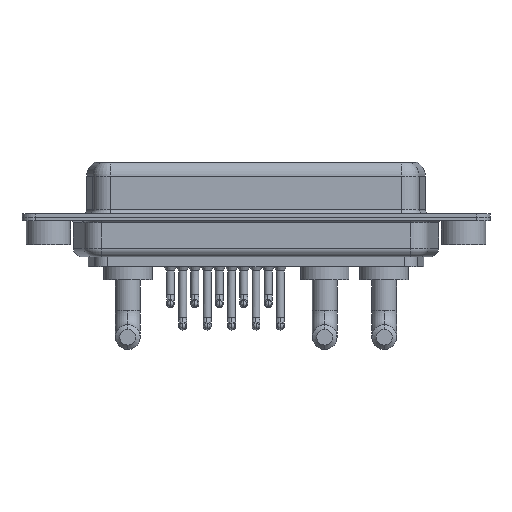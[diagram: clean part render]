
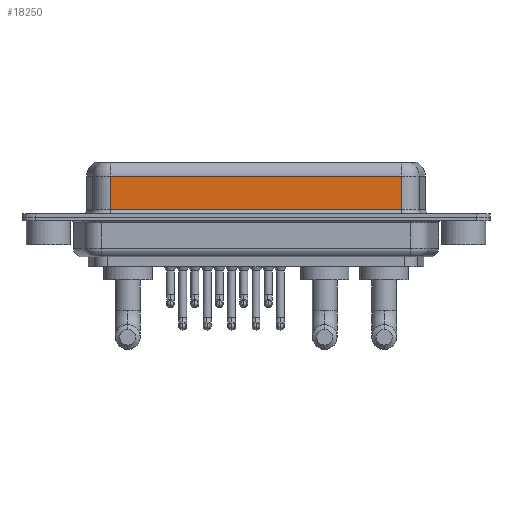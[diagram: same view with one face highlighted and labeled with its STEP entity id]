
A CAD part, front view. The second image highlights one B-rep face of the part: STEP entity #18250.
In plain terms, the highlighted planar face has unit normal (0, -1, 0).
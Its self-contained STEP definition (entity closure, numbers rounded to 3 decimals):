
#983 = EDGE_CURVE ( 'NONE', #9969, #15466, #7790, .T. ) ;
#1266 = CARTESIAN_POINT ( 'NONE',  ( 7.013, -3.95, 0.9 ) ) ;
#2464 = LINE ( 'NONE', #8373, #13477 ) ;
#3045 = DIRECTION ( 'NONE',  ( 0., 1., 0. ) ) ;
#3876 = ORIENTED_EDGE ( 'NONE', *, *, #6217, .T. ) ;
#4657 = VECTOR ( 'NONE', #13646, 1000. ) ;
#5276 = CARTESIAN_POINT ( 'NONE',  ( 40.037, -3.95, 4.65 ) ) ;
#6217 = EDGE_CURVE ( 'NONE', #8780, #9969, #9509, .T. ) ;
#6333 = VERTEX_POINT ( 'NONE', #12766 ) ;
#6337 = CARTESIAN_POINT ( 'NONE',  ( 7.013, -3.95, 6.4 ) ) ;
#6351 = CARTESIAN_POINT ( 'NONE',  ( 7.013, -3.95, 4.65 ) ) ;
#7225 = VECTOR ( 'NONE', #15388, 1000. ) ;
#7760 = DIRECTION ( 'NONE',  ( 0., 0., -1. ) ) ;
#7790 = LINE ( 'NONE', #6337, #4657 ) ;
#8373 = CARTESIAN_POINT ( 'NONE',  ( 40.037, -3.95, 0.9 ) ) ;
#8780 = VERTEX_POINT ( 'NONE', #5276 ) ;
#8953 = DIRECTION ( 'NONE',  ( 0., 0., 1. ) ) ;
#9008 = LINE ( 'NONE', #10661, #13821 ) ;
#9509 = LINE ( 'NONE', #15669, #7225 ) ;
#9810 = DIRECTION ( 'NONE',  ( 1., 0., 0. ) ) ;
#9969 = VERTEX_POINT ( 'NONE', #6351 ) ;
#10257 = AXIS2_PLACEMENT_3D ( 'NONE', #14534, #3045, #8953 ) ;
#10329 = ORIENTED_EDGE ( 'NONE', *, *, #12552, .F. ) ;
#10661 = CARTESIAN_POINT ( 'NONE',  ( 40.037, -3.95, 6.4 ) ) ;
#11370 = EDGE_CURVE ( 'NONE', #15466, #6333, #2464, .T. ) ;
#11758 = ORIENTED_EDGE ( 'NONE', *, *, #983, .T. ) ;
#12519 = ORIENTED_EDGE ( 'NONE', *, *, #11370, .T. ) ;
#12552 = EDGE_CURVE ( 'NONE', #8780, #6333, #9008, .T. ) ;
#12766 = CARTESIAN_POINT ( 'NONE',  ( 40.037, -3.95, 0.9 ) ) ;
#13477 = VECTOR ( 'NONE', #9810, 1000. ) ;
#13646 = DIRECTION ( 'NONE',  ( 0., 0., -1. ) ) ;
#13821 = VECTOR ( 'NONE', #7760, 1000. ) ;
#14534 = CARTESIAN_POINT ( 'NONE',  ( 40.037, -3.95, 6.4 ) ) ;
#15388 = DIRECTION ( 'NONE',  ( -1., 0., 0. ) ) ;
#15466 = VERTEX_POINT ( 'NONE', #1266 ) ;
#15669 = CARTESIAN_POINT ( 'NONE',  ( 40.037, -3.95, 4.65 ) ) ;
#16284 = PLANE ( 'NONE',  #10257 ) ;
#16487 = FACE_OUTER_BOUND ( 'NONE', #18064, .T. ) ;
#18064 = EDGE_LOOP ( 'NONE', ( #10329, #3876, #11758, #12519 ) ) ;
#18250 = ADVANCED_FACE ( 'NONE', ( #16487 ), #16284, .F. ) ;
